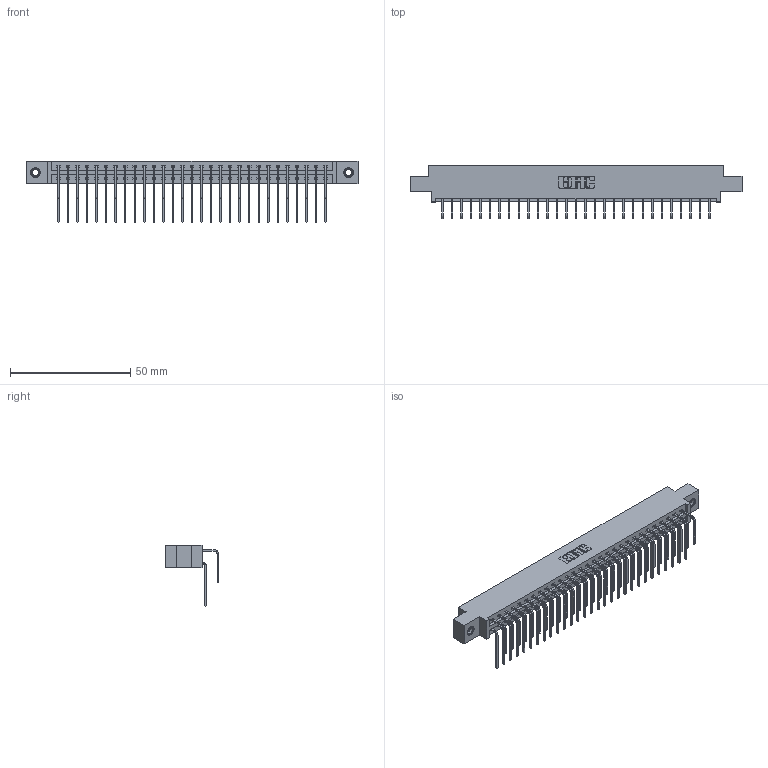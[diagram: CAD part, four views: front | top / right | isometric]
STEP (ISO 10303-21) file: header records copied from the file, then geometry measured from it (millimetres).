
FILE_DESCRIPTION (( 'STEP AP203' ), '1' );
FILE_NAME ('337-058-558-807.STEP', '2019-10-11T21:05:14', ( '' ), ( '' ), 'SwSTEP 2.0', 'SolidWorks 2016', '' );
FILE_SCHEMA (( 'CONFIG_CONTROL_DESIGN' ));
Length unit declared in the file: inch
Products named in the file (5): 337 Part_0.170 Offset - 0.156 Dia-TI; 345-292-001_558 Tail - 2; 345-250-001_345-250-005-103; 345-292-001_558 559 Tail - 1; 337-058-558-807
Assembly tree (61 placements, depth 2):
  337-058-558-807
    337 Part_0.170 Offset - 0.156 Dia-TI
    345-292-001_558 559 Tail - 1  x29
    345-292-001_558 Tail - 2  x29
    345-250-001_345-250-005-103  x2
Bounding box: 137.92 x 22.17 x 25.53 mm (x, y, z)
Volume: 14565.8 mm3; surface area: 18164.2 mm2
Topology: 61 solids, 61 shells, 3426 faces, 10145 edges, 6678 vertices
Faces by surface type: plane 2426, cylinder 984, cone 12, torus 4
Entity records: 27268 total; most frequent: CARTESIAN_POINT 4632, ORIENTED_EDGE 4510, DIRECTION 3977, EDGE_CURVE 2255, LINE 2067, VECTOR 2067, VERTEX_POINT 1496, AXIS2_PLACEMENT_3D 955
